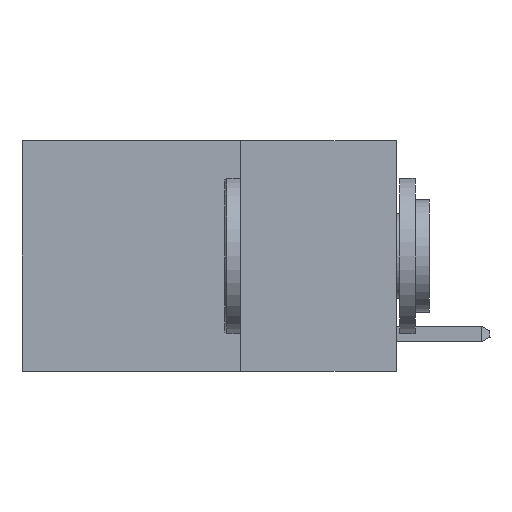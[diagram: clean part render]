
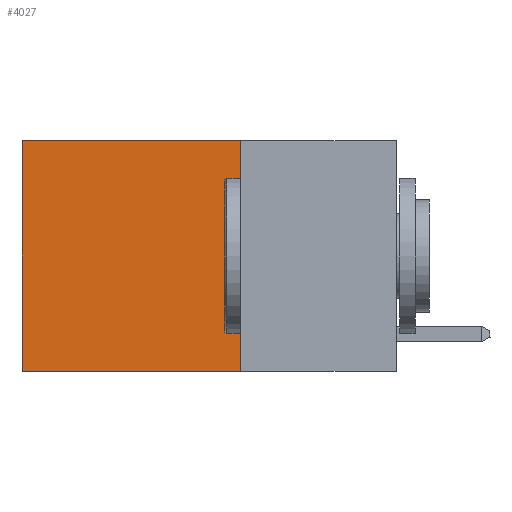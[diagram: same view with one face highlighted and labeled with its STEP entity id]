
A CAD part, left-side view. The second image highlights one B-rep face of the part: STEP entity #4027.
In plain terms, the highlighted planar face has unit normal (-1, 0, 0).
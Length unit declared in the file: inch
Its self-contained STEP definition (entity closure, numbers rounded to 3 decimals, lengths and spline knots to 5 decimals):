
#270 = DIRECTION ( 'NONE',  ( 0., 1., 0. ) ) ;
#561 = CARTESIAN_POINT ( 'NONE',  ( 0.2625, 0.25, 0. ) ) ;
#692 = ORIENTED_EDGE ( 'NONE', *, *, #8664, .T. ) ;
#1260 = CARTESIAN_POINT ( 'NONE',  ( 0.2625, 0.6, -0.37 ) ) ;
#1667 = LINE ( 'NONE', #18717, #4401 ) ;
#1769 = DIRECTION ( 'NONE',  ( 0., 0., -1. ) ) ;
#4027 = ADVANCED_FACE ( 'NONE', ( #14680 ), #13884, .F. ) ;
#4077 = ORIENTED_EDGE ( 'NONE', *, *, #15873, .T. ) ;
#4209 = CARTESIAN_POINT ( 'NONE',  ( 0.2625, 0.25, 0. ) ) ;
#4401 = VECTOR ( 'NONE', #1769, 39.37008 ) ;
#5743 = CARTESIAN_POINT ( 'NONE',  ( 0.2625, 0.6, 0. ) ) ;
#6155 = ORIENTED_EDGE ( 'NONE', *, *, #20112, .F. ) ;
#7082 = VERTEX_POINT ( 'NONE', #1260 ) ;
#7703 = VECTOR ( 'NONE', #11396, 39.37008 ) ;
#7822 = LINE ( 'NONE', #4209, #21400 ) ;
#8353 = VERTEX_POINT ( 'NONE', #561 ) ;
#8512 = LINE ( 'NONE', #8617, #18433 ) ;
#8617 = CARTESIAN_POINT ( 'NONE',  ( 0.2625, 0.25, 0. ) ) ;
#8664 = EDGE_CURVE ( 'NONE', #19393, #7082, #1667, .T. ) ;
#9408 = DIRECTION ( 'NONE',  ( 0., 0., -1. ) ) ;
#9713 = CARTESIAN_POINT ( 'NONE',  ( 0.2625, 0.25, -0.37 ) ) ;
#10880 = AXIS2_PLACEMENT_3D ( 'NONE', #19188, #18860, #11956 ) ;
#11396 = DIRECTION ( 'NONE',  ( 0., 1., 0. ) ) ;
#11433 = ORIENTED_EDGE ( 'NONE', *, *, #18662, .F. ) ;
#11956 = DIRECTION ( 'NONE',  ( 0., 0., -1. ) ) ;
#13099 = LINE ( 'NONE', #9713, #7703 ) ;
#13435 = CARTESIAN_POINT ( 'NONE',  ( 0.2625, 0.25, -0.37 ) ) ;
#13776 = VERTEX_POINT ( 'NONE', #13435 ) ;
#13884 = PLANE ( 'NONE',  #10880 ) ;
#14680 = FACE_OUTER_BOUND ( 'NONE', #21401, .T. ) ;
#15873 = EDGE_CURVE ( 'NONE', #8353, #19393, #8512, .T. ) ;
#18433 = VECTOR ( 'NONE', #270, 39.37008 ) ;
#18662 = EDGE_CURVE ( 'NONE', #8353, #13776, #7822, .T. ) ;
#18717 = CARTESIAN_POINT ( 'NONE',  ( 0.2625, 0.6, 0. ) ) ;
#18860 = DIRECTION ( 'NONE',  ( 1., 0., 0. ) ) ;
#19188 = CARTESIAN_POINT ( 'NONE',  ( 0.2625, 0.25, 0. ) ) ;
#19393 = VERTEX_POINT ( 'NONE', #5743 ) ;
#20112 = EDGE_CURVE ( 'NONE', #13776, #7082, #13099, .T. ) ;
#21400 = VECTOR ( 'NONE', #9408, 39.37008 ) ;
#21401 = EDGE_LOOP ( 'NONE', ( #692, #6155, #11433, #4077 ) ) ;
